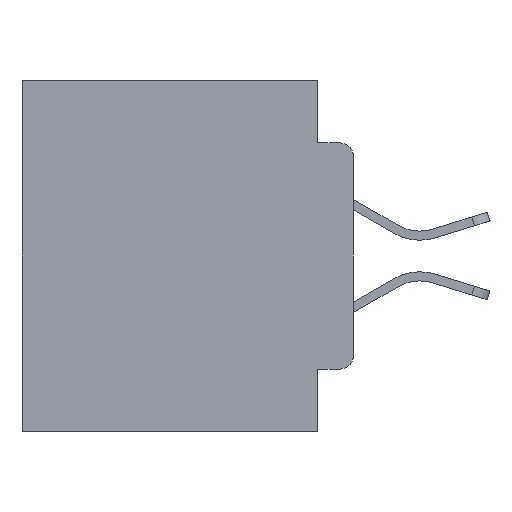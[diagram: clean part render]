
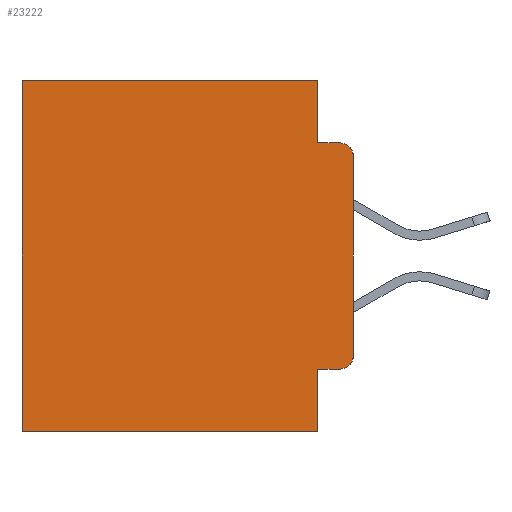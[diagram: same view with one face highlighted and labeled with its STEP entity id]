
A CAD part, left-side view. The second image highlights one B-rep face of the part: STEP entity #23222.
In plain terms, the highlighted planar face has unit normal (-1, 0, 0).
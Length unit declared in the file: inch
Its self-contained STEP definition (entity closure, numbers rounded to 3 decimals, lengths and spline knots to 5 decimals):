
#219 = ORIENTED_EDGE ( 'NONE', *, *, #16542, .T. ) ;
#258 = LINE ( 'NONE', #20616, #17018 ) ;
#870 = EDGE_CURVE ( 'NONE', #10615, #14501, #26317, .T. ) ;
#1061 = CARTESIAN_POINT ( 'NONE',  ( 0.298, 0.051, 0. ) ) ;
#1440 = DIRECTION ( 'NONE',  ( 0., -1., 0. ) ) ;
#1753 = CARTESIAN_POINT ( 'NONE',  ( 0.298, 0.02, -0.4115 ) ) ;
#2312 = EDGE_CURVE ( 'NONE', #14501, #20484, #6574, .T. ) ;
#3108 = ORIENTED_EDGE ( 'NONE', *, *, #870, .F. ) ;
#3211 = ORIENTED_EDGE ( 'NONE', *, *, #22845, .T. ) ;
#3508 = CARTESIAN_POINT ( 'NONE',  ( 0.298, 0.051, 0. ) ) ;
#3564 = DIRECTION ( 'NONE',  ( 0., 1., 0. ) ) ;
#4516 = VERTEX_POINT ( 'NONE', #8069 ) ;
#4748 = CIRCLE ( 'NONE', #25077, 0.02 ) ;
#4936 = VECTOR ( 'NONE', #25541, 39.37008 ) ;
#5222 = VERTEX_POINT ( 'NONE', #6758 ) ;
#5437 = LINE ( 'NONE', #16151, #16267 ) ;
#6194 = VERTEX_POINT ( 'NONE', #18497 ) ;
#6574 = LINE ( 'NONE', #27201, #27538 ) ;
#6758 = CARTESIAN_POINT ( 'NONE',  ( 0.298, 0., -0.3915 ) ) ;
#7111 = CARTESIAN_POINT ( 'NONE',  ( 0.298, 0.473, -0.5 ) ) ;
#7247 = CARTESIAN_POINT ( 'NONE',  ( 0.298, 0.02, -0.3915 ) ) ;
#7349 = CARTESIAN_POINT ( 'NONE',  ( 0.298, 0.051, -0.4115 ) ) ;
#7505 = VECTOR ( 'NONE', #15792, 39.37008 ) ;
#7612 = DIRECTION ( 'NONE',  ( -1., 0., 0. ) ) ;
#8069 = CARTESIAN_POINT ( 'NONE',  ( 0.298, 0.051, -0.0885 ) ) ;
#8682 = EDGE_CURVE ( 'NONE', #9920, #4516, #13345, .T. ) ;
#8896 = FACE_OUTER_BOUND ( 'NONE', #12192, .T. ) ;
#9211 = CARTESIAN_POINT ( 'NONE',  ( 0.298, 0.051, -0.4115 ) ) ;
#9446 = DIRECTION ( 'NONE',  ( 0., 0., -1. ) ) ;
#9716 = EDGE_CURVE ( 'NONE', #16647, #5222, #4748, .T. ) ;
#9920 = VERTEX_POINT ( 'NONE', #3508 ) ;
#10615 = VERTEX_POINT ( 'NONE', #7349 ) ;
#10932 = VECTOR ( 'NONE', #1440, 39.37008 ) ;
#11564 = EDGE_CURVE ( 'NONE', #19436, #5222, #16427, .T. ) ;
#11598 = LINE ( 'NONE', #26854, #10932 ) ;
#11738 = ORIENTED_EDGE ( 'NONE', *, *, #18458, .F. ) ;
#12179 = DIRECTION ( 'NONE',  ( 0., 0., -1. ) ) ;
#12192 = EDGE_LOOP ( 'NONE', ( #16196, #3211, #11738, #26390, #219, #23484, #23205, #3108, #25786, #27051 ) ) ;
#12751 = CARTESIAN_POINT ( 'NONE',  ( 0.298, 0.02, -0.0885 ) ) ;
#13322 = DIRECTION ( 'NONE',  ( 0., 0., -1. ) ) ;
#13345 = LINE ( 'NONE', #1061, #23631 ) ;
#13889 = VERTEX_POINT ( 'NONE', #12751 ) ;
#13972 = LINE ( 'NONE', #9211, #7505 ) ;
#14501 = VERTEX_POINT ( 'NONE', #25036 ) ;
#14803 = VECTOR ( 'NONE', #25136, 39.37008 ) ;
#15351 = CARTESIAN_POINT ( 'NONE',  ( 0.298, 0., 0. ) ) ;
#15792 = DIRECTION ( 'NONE',  ( 0., -1., 0. ) ) ;
#16051 = CARTESIAN_POINT ( 'NONE',  ( 0.298, 0.051, 0. ) ) ;
#16151 = CARTESIAN_POINT ( 'NONE',  ( 0.298, 0.473, 0. ) ) ;
#16196 = ORIENTED_EDGE ( 'NONE', *, *, #11564, .F. ) ;
#16267 = VECTOR ( 'NONE', #18227, 39.37008 ) ;
#16427 = LINE ( 'NONE', #21435, #4936 ) ;
#16542 = EDGE_CURVE ( 'NONE', #9920, #6194, #258, .T. ) ;
#16647 = VERTEX_POINT ( 'NONE', #1753 ) ;
#17018 = VECTOR ( 'NONE', #3564, 39.37008 ) ;
#17128 = AXIS2_PLACEMENT_3D ( 'NONE', #15351, #25621, #13322 ) ;
#18176 = EDGE_CURVE ( 'NONE', #10615, #16647, #13972, .T. ) ;
#18227 = DIRECTION ( 'NONE',  ( 0., 0., -1. ) ) ;
#18295 = EDGE_CURVE ( 'NONE', #6194, #20484, #5437, .T. ) ;
#18458 = EDGE_CURVE ( 'NONE', #4516, #13889, #11598, .T. ) ;
#18497 = CARTESIAN_POINT ( 'NONE',  ( 0.298, 0.473, 0. ) ) ;
#19436 = VERTEX_POINT ( 'NONE', #22079 ) ;
#20289 = CARTESIAN_POINT ( 'NONE',  ( 0.298, 0.02, -0.1085 ) ) ;
#20484 = VERTEX_POINT ( 'NONE', #7111 ) ;
#20616 = CARTESIAN_POINT ( 'NONE',  ( 0.298, 0., 0. ) ) ;
#21435 = CARTESIAN_POINT ( 'NONE',  ( 0.298, 0., 0. ) ) ;
#21994 = DIRECTION ( 'NONE',  ( -1., 0., 0. ) ) ;
#22079 = CARTESIAN_POINT ( 'NONE',  ( 0.298, 0., -0.1085 ) ) ;
#22331 = DIRECTION ( 'NONE',  ( 0., 0., -1. ) ) ;
#22845 = EDGE_CURVE ( 'NONE', #19436, #13889, #23011, .T. ) ;
#23011 = CIRCLE ( 'NONE', #24587, 0.02 ) ;
#23205 = ORIENTED_EDGE ( 'NONE', *, *, #2312, .F. ) ;
#23222 = ADVANCED_FACE ( 'NONE', ( #8896 ), #23563, .F. ) ;
#23484 = ORIENTED_EDGE ( 'NONE', *, *, #18295, .T. ) ;
#23563 = PLANE ( 'NONE',  #17128 ) ;
#23631 = VECTOR ( 'NONE', #12179, 39.37008 ) ;
#24587 = AXIS2_PLACEMENT_3D ( 'NONE', #20289, #7612, #22331 ) ;
#25036 = CARTESIAN_POINT ( 'NONE',  ( 0.298, 0.051, -0.5 ) ) ;
#25077 = AXIS2_PLACEMENT_3D ( 'NONE', #7247, #21994, #9446 ) ;
#25136 = DIRECTION ( 'NONE',  ( 0., 0., -1. ) ) ;
#25541 = DIRECTION ( 'NONE',  ( 0., 0., -1. ) ) ;
#25621 = DIRECTION ( 'NONE',  ( 1., 0., 0. ) ) ;
#25786 = ORIENTED_EDGE ( 'NONE', *, *, #18176, .T. ) ;
#25841 = DIRECTION ( 'NONE',  ( 0., 1., 0. ) ) ;
#26317 = LINE ( 'NONE', #16051, #14803 ) ;
#26390 = ORIENTED_EDGE ( 'NONE', *, *, #8682, .F. ) ;
#26854 = CARTESIAN_POINT ( 'NONE',  ( 0.298, 0.051, -0.0885 ) ) ;
#27051 = ORIENTED_EDGE ( 'NONE', *, *, #9716, .T. ) ;
#27201 = CARTESIAN_POINT ( 'NONE',  ( 0.298, 0., -0.5 ) ) ;
#27538 = VECTOR ( 'NONE', #25841, 39.37008 ) ;
